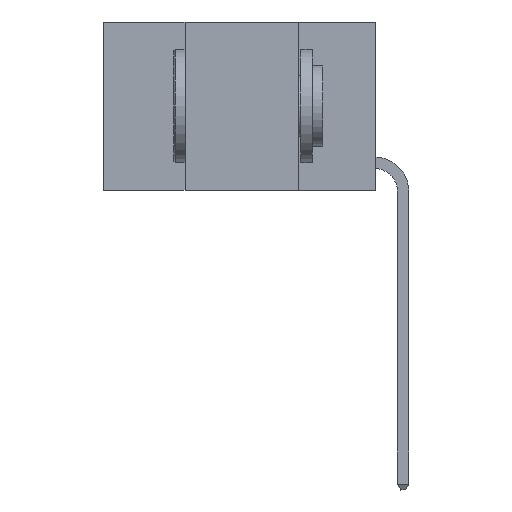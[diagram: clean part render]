
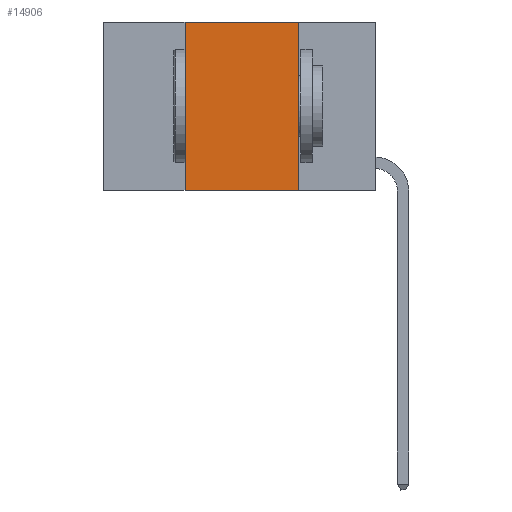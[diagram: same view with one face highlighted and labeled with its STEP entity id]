
A CAD part, left-side view. The second image highlights one B-rep face of the part: STEP entity #14906.
In plain terms, the highlighted planar face has unit normal (-1, 0, 0).
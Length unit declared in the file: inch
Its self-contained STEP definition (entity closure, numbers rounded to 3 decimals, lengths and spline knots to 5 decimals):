
#37 = DIRECTION ( 'NONE',  ( 0., 0., -1. ) ) ;
#610 = VERTEX_POINT ( 'NONE', #12247 ) ;
#779 = VECTOR ( 'NONE', #3960, 39.37008 ) ;
#1298 = EDGE_LOOP ( 'NONE', ( #4546, #4645, #4676, #4850 ) ) ;
#1518 = LINE ( 'NONE', #13692, #11346 ) ;
#1889 = VECTOR ( 'NONE', #6312, 39.37008 ) ;
#2384 = FACE_OUTER_BOUND ( 'NONE', #1298, .T. ) ;
#2738 = DIRECTION ( 'NONE',  ( 1., 0., 0. ) ) ;
#3029 = EDGE_CURVE ( 'NONE', #6511, #9747, #14343, .T. ) ;
#3960 = DIRECTION ( 'NONE',  ( 0., 0., 1. ) ) ;
#4546 = ORIENTED_EDGE ( 'NONE', *, *, #9478, .F. ) ;
#4645 = ORIENTED_EDGE ( 'NONE', *, *, #3029, .F. ) ;
#4676 = ORIENTED_EDGE ( 'NONE', *, *, #10293, .F. ) ;
#4830 = VECTOR ( 'NONE', #13373, 39.37008 ) ;
#4850 = ORIENTED_EDGE ( 'NONE', *, *, #14965, .T. ) ;
#5082 = CARTESIAN_POINT ( 'NONE',  ( 0., 0.17, 0. ) ) ;
#5502 = CARTESIAN_POINT ( 'NONE',  ( 0., 0.42, 0. ) ) ;
#6312 = DIRECTION ( 'NONE',  ( 0., 0., -1. ) ) ;
#6460 = CARTESIAN_POINT ( 'NONE',  ( 0., 0.6, 0. ) ) ;
#6511 = VERTEX_POINT ( 'NONE', #5502 ) ;
#6557 = DIRECTION ( 'NONE',  ( 0., -1., 0. ) ) ;
#6880 = AXIS2_PLACEMENT_3D ( 'NONE', #6460, #2738, #37 ) ;
#7503 = LINE ( 'NONE', #10056, #779 ) ;
#7678 = PLANE ( 'NONE',  #6880 ) ;
#7705 = LINE ( 'NONE', #5082, #1889 ) ;
#9137 = CARTESIAN_POINT ( 'NONE',  ( 0., 0.17, 0. ) ) ;
#9478 = EDGE_CURVE ( 'NONE', #9747, #10762, #7705, .T. ) ;
#9747 = VERTEX_POINT ( 'NONE', #9137 ) ;
#10056 = CARTESIAN_POINT ( 'NONE',  ( 0., 0.42, 0. ) ) ;
#10293 = EDGE_CURVE ( 'NONE', #610, #6511, #7503, .T. ) ;
#10762 = VERTEX_POINT ( 'NONE', #12075 ) ;
#11346 = VECTOR ( 'NONE', #6557, 39.37008 ) ;
#12075 = CARTESIAN_POINT ( 'NONE',  ( 0., 0.17, -0.37 ) ) ;
#12196 = CARTESIAN_POINT ( 'NONE',  ( 0., 0.6, 0. ) ) ;
#12247 = CARTESIAN_POINT ( 'NONE',  ( 0., 0.42, -0.37 ) ) ;
#13373 = DIRECTION ( 'NONE',  ( 0., -1., 0. ) ) ;
#13692 = CARTESIAN_POINT ( 'NONE',  ( 0., 0.6, -0.37 ) ) ;
#14343 = LINE ( 'NONE', #12196, #4830 ) ;
#14906 = ADVANCED_FACE ( 'NONE', ( #2384 ), #7678, .F. ) ;
#14965 = EDGE_CURVE ( 'NONE', #610, #10762, #1518, .T. ) ;
